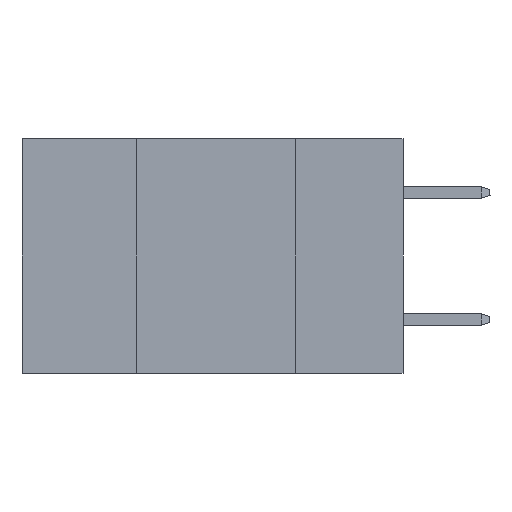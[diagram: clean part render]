
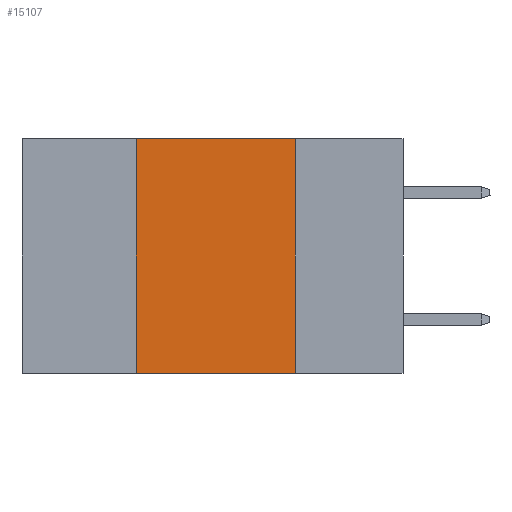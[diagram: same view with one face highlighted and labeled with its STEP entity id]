
A CAD part, left-side view. The second image highlights one B-rep face of the part: STEP entity #15107.
In plain terms, the highlighted planar face has unit normal (-1, 0, 0).
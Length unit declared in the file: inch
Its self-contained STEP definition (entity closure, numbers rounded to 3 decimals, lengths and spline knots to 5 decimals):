
#1241 = CARTESIAN_POINT ( 'NONE',  ( 0., 0.6, 0. ) ) ;
#3281 = CARTESIAN_POINT ( 'NONE',  ( 0., 0.42, -0.37 ) ) ;
#3436 = EDGE_CURVE ( 'NONE', #20853, #29166, #26358, .T. ) ;
#3714 = DIRECTION ( 'NONE',  ( 1., 0., 0. ) ) ;
#3735 = ORIENTED_EDGE ( 'NONE', *, *, #3436, .T. ) ;
#4301 = CARTESIAN_POINT ( 'NONE',  ( 0., 0.6, -0.37 ) ) ;
#4568 = VERTEX_POINT ( 'NONE', #34353 ) ;
#5293 = EDGE_CURVE ( 'NONE', #4568, #29166, #15360, .T. ) ;
#6385 = FACE_OUTER_BOUND ( 'NONE', #15004, .T. ) ;
#6862 = CARTESIAN_POINT ( 'NONE',  ( 0., 0.17, -0.37 ) ) ;
#15004 = EDGE_LOOP ( 'NONE', ( #15988, #25551, #31945, #3735 ) ) ;
#15107 = ADVANCED_FACE ( 'NONE', ( #6385 ), #17228, .F. ) ;
#15360 = LINE ( 'NONE', #15711, #23132 ) ;
#15711 = CARTESIAN_POINT ( 'NONE',  ( 0., 0.17, 0. ) ) ;
#15988 = ORIENTED_EDGE ( 'NONE', *, *, #5293, .F. ) ;
#16459 = CARTESIAN_POINT ( 'NONE',  ( 0., 0.6, 0. ) ) ;
#16661 = CARTESIAN_POINT ( 'NONE',  ( 0., 0.42, 0. ) ) ;
#17228 = PLANE ( 'NONE',  #19283 ) ;
#19283 = AXIS2_PLACEMENT_3D ( 'NONE', #1241, #3714, #25059 ) ;
#19300 = CARTESIAN_POINT ( 'NONE',  ( 0., 0.42, 0. ) ) ;
#20853 = VERTEX_POINT ( 'NONE', #3281 ) ;
#21763 = LINE ( 'NONE', #16459, #22702 ) ;
#22702 = VECTOR ( 'NONE', #30504, 39.37008 ) ;
#23132 = VECTOR ( 'NONE', #26204, 39.37008 ) ;
#23138 = DIRECTION ( 'NONE',  ( 0., -1., 0. ) ) ;
#23942 = DIRECTION ( 'NONE',  ( 0., 0., 1. ) ) ;
#25059 = DIRECTION ( 'NONE',  ( 0., 0., -1. ) ) ;
#25404 = VECTOR ( 'NONE', #23138, 39.37008 ) ;
#25551 = ORIENTED_EDGE ( 'NONE', *, *, #34643, .F. ) ;
#26204 = DIRECTION ( 'NONE',  ( 0., 0., -1. ) ) ;
#26358 = LINE ( 'NONE', #4301, #25404 ) ;
#27329 = LINE ( 'NONE', #16661, #29465 ) ;
#29166 = VERTEX_POINT ( 'NONE', #6862 ) ;
#29465 = VECTOR ( 'NONE', #23942, 39.37008 ) ;
#30504 = DIRECTION ( 'NONE',  ( 0., -1., 0. ) ) ;
#30774 = VERTEX_POINT ( 'NONE', #19300 ) ;
#30788 = EDGE_CURVE ( 'NONE', #20853, #30774, #27329, .T. ) ;
#31945 = ORIENTED_EDGE ( 'NONE', *, *, #30788, .F. ) ;
#34353 = CARTESIAN_POINT ( 'NONE',  ( 0., 0.17, 0. ) ) ;
#34643 = EDGE_CURVE ( 'NONE', #30774, #4568, #21763, .T. ) ;
